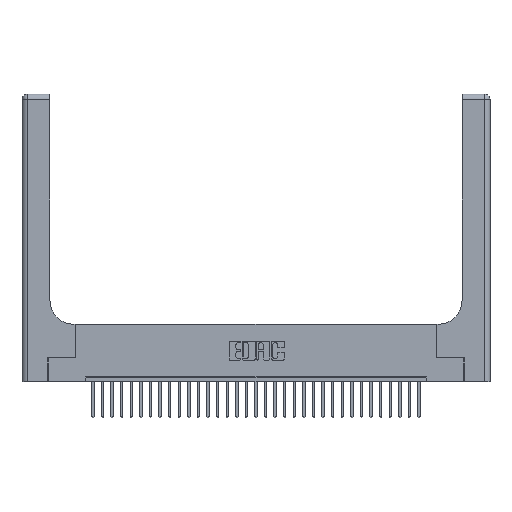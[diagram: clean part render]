
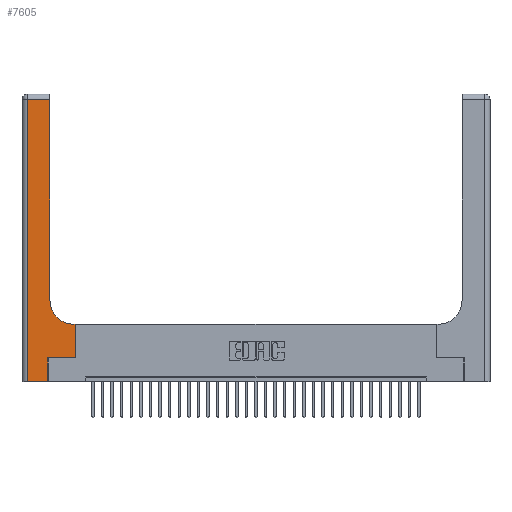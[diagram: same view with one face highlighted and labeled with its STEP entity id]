
A CAD part, top view. The second image highlights one B-rep face of the part: STEP entity #7605.
In plain terms, the highlighted planar face has unit normal (0, 0, 1).
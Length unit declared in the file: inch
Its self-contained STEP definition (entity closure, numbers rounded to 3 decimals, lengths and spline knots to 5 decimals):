
#213 = ORIENTED_EDGE ( 'NONE', *, *, #30975, .T. ) ;
#949 = EDGE_LOOP ( 'NONE', ( #30456, #7041, #7508, #29195, #213, #12581, #7229, #5280, #1961 ) ) ;
#973 = VERTEX_POINT ( 'NONE', #20397 ) ;
#1961 = ORIENTED_EDGE ( 'NONE', *, *, #5189, .T. ) ;
#2016 = CARTESIAN_POINT ( 'NONE',  ( 0., 0., 0.37 ) ) ;
#3442 = CARTESIAN_POINT ( 'NONE',  ( 0.06, 2.94, 0.37 ) ) ;
#3736 = VECTOR ( 'NONE', #12718, 39.37008 ) ;
#4030 = LINE ( 'NONE', #19105, #9501 ) ;
#4143 = CARTESIAN_POINT ( 'NONE',  ( 0.5585, 0.25, 0.37 ) ) ;
#4608 = CARTESIAN_POINT ( 'NONE',  ( 0.269, 0., 0.37 ) ) ;
#5167 = CARTESIAN_POINT ( 'NONE',  ( 0.2915, 3., 0.37 ) ) ;
#5189 = EDGE_CURVE ( 'NONE', #30376, #27866, #23418, .T. ) ;
#5280 = ORIENTED_EDGE ( 'NONE', *, *, #6829, .T. ) ;
#5964 = CARTESIAN_POINT ( 'NONE',  ( 0.2915, 0.85, 0.37 ) ) ;
#6222 = VERTEX_POINT ( 'NONE', #7452 ) ;
#6605 = VERTEX_POINT ( 'NONE', #29254 ) ;
#6829 = EDGE_CURVE ( 'NONE', #8728, #30376, #19486, .T. ) ;
#7041 = ORIENTED_EDGE ( 'NONE', *, *, #23340, .T. ) ;
#7087 = EDGE_CURVE ( 'NONE', #6605, #8728, #20621, .T. ) ;
#7229 = ORIENTED_EDGE ( 'NONE', *, *, #7087, .T. ) ;
#7452 = CARTESIAN_POINT ( 'NONE',  ( 0.2915, 2.94, 0.37 ) ) ;
#7508 = ORIENTED_EDGE ( 'NONE', *, *, #13657, .T. ) ;
#7605 = ADVANCED_FACE ( 'NONE', ( #30064 ), #18462, .F. ) ;
#8483 = VECTOR ( 'NONE', #13977, 39.37008 ) ;
#8645 = VERTEX_POINT ( 'NONE', #27000 ) ;
#8728 = VERTEX_POINT ( 'NONE', #21223 ) ;
#9501 = VECTOR ( 'NONE', #23727, 39.37008 ) ;
#9851 = LINE ( 'NONE', #4608, #32254 ) ;
#10718 = VERTEX_POINT ( 'NONE', #15858 ) ;
#10833 = LINE ( 'NONE', #29141, #8483 ) ;
#11092 = CARTESIAN_POINT ( 'NONE',  ( 0., 3., 0.37 ) ) ;
#12043 = DIRECTION ( 'NONE',  ( 0., 1., 0. ) ) ;
#12490 = VERTEX_POINT ( 'NONE', #3442 ) ;
#12581 = ORIENTED_EDGE ( 'NONE', *, *, #20202, .T. ) ;
#12718 = DIRECTION ( 'NONE',  ( 1., 0., 0. ) ) ;
#13604 = DIRECTION ( 'NONE',  ( -1., 0., 0. ) ) ;
#13657 = EDGE_CURVE ( 'NONE', #12490, #10718, #18035, .T. ) ;
#13977 = DIRECTION ( 'NONE',  ( 1., 0., 0. ) ) ;
#14280 = CARTESIAN_POINT ( 'NONE',  ( 0.06, 3., 0.37 ) ) ;
#14611 = VECTOR ( 'NONE', #17571, 39.37008 ) ;
#15858 = CARTESIAN_POINT ( 'NONE',  ( 0.06, 0., 0.37 ) ) ;
#16336 = EDGE_CURVE ( 'NONE', #10718, #973, #17470, .T. ) ;
#16468 = VECTOR ( 'NONE', #32075, 39.37008 ) ;
#16487 = AXIS2_PLACEMENT_3D ( 'NONE', #27316, #30053, #32392 ) ;
#17451 = EDGE_CURVE ( 'NONE', #27866, #6222, #18951, .T. ) ;
#17470 = LINE ( 'NONE', #2016, #3736 ) ;
#17571 = DIRECTION ( 'NONE',  ( 0., 1., 0. ) ) ;
#18035 = LINE ( 'NONE', #14280, #16468 ) ;
#18462 = PLANE ( 'NONE',  #27419 ) ;
#18951 = LINE ( 'NONE', #5167, #14611 ) ;
#19105 = CARTESIAN_POINT ( 'NONE',  ( 0., 2.94, 0.37 ) ) ;
#19486 = LINE ( 'NONE', #20671, #29283 ) ;
#20202 = EDGE_CURVE ( 'NONE', #8645, #6605, #10833, .T. ) ;
#20397 = CARTESIAN_POINT ( 'NONE',  ( 0.269, 0., 0.37 ) ) ;
#20621 = LINE ( 'NONE', #4143, #21427 ) ;
#20671 = CARTESIAN_POINT ( 'NONE',  ( 0.2915, 0.6, 0.37 ) ) ;
#21223 = CARTESIAN_POINT ( 'NONE',  ( 0.5585, 0.6, 0.37 ) ) ;
#21427 = VECTOR ( 'NONE', #26846, 39.37008 ) ;
#23340 = EDGE_CURVE ( 'NONE', #6222, #12490, #4030, .T. ) ;
#23418 = CIRCLE ( 'NONE', #16487, 0.25 ) ;
#23727 = DIRECTION ( 'NONE',  ( -1., 0., 0. ) ) ;
#23926 = DIRECTION ( 'NONE',  ( -1., 0., 0. ) ) ;
#25785 = DIRECTION ( 'NONE',  ( 0., 0., -1. ) ) ;
#26846 = DIRECTION ( 'NONE',  ( 0., 1., 0. ) ) ;
#27000 = CARTESIAN_POINT ( 'NONE',  ( 0.269, 0.25, 0.37 ) ) ;
#27316 = CARTESIAN_POINT ( 'NONE',  ( 0.5415, 0.85, 0.37 ) ) ;
#27419 = AXIS2_PLACEMENT_3D ( 'NONE', #11092, #25785, #13604 ) ;
#27866 = VERTEX_POINT ( 'NONE', #5964 ) ;
#29141 = CARTESIAN_POINT ( 'NONE',  ( 0.269, 0.25, 0.37 ) ) ;
#29195 = ORIENTED_EDGE ( 'NONE', *, *, #16336, .T. ) ;
#29254 = CARTESIAN_POINT ( 'NONE',  ( 0.5585, 0.25, 0.37 ) ) ;
#29283 = VECTOR ( 'NONE', #23926, 39.37008 ) ;
#30053 = DIRECTION ( 'NONE',  ( 0., 0., -1. ) ) ;
#30064 = FACE_OUTER_BOUND ( 'NONE', #949, .T. ) ;
#30376 = VERTEX_POINT ( 'NONE', #31515 ) ;
#30456 = ORIENTED_EDGE ( 'NONE', *, *, #17451, .T. ) ;
#30975 = EDGE_CURVE ( 'NONE', #973, #8645, #9851, .T. ) ;
#31515 = CARTESIAN_POINT ( 'NONE',  ( 0.5415, 0.6, 0.37 ) ) ;
#32075 = DIRECTION ( 'NONE',  ( 0., -1., 0. ) ) ;
#32254 = VECTOR ( 'NONE', #12043, 39.37008 ) ;
#32392 = DIRECTION ( 'NONE',  ( 1., 0., 0. ) ) ;
